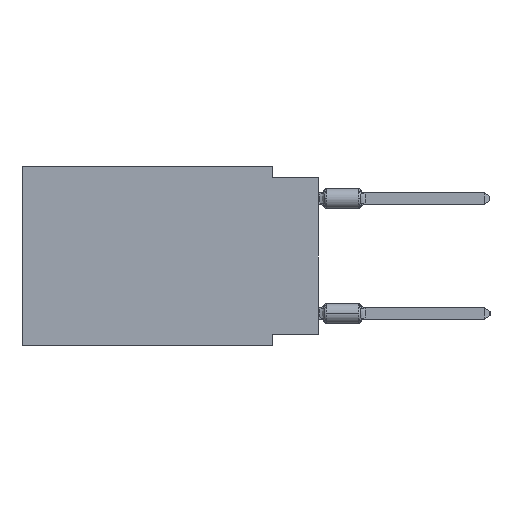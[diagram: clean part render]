
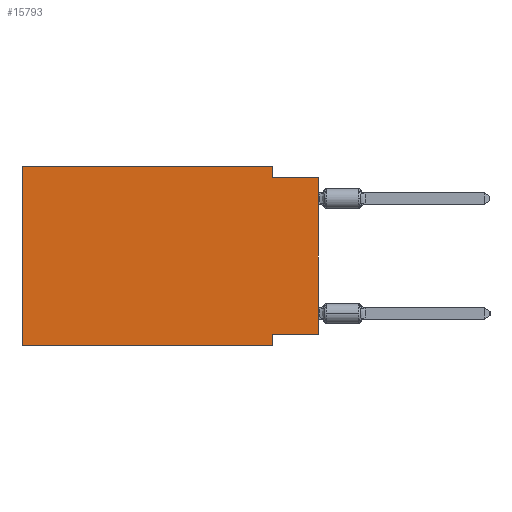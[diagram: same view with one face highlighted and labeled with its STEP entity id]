
A CAD part, left-side view. The second image highlights one B-rep face of the part: STEP entity #15793.
In plain terms, the highlighted planar face has unit normal (-1, 0, 0).
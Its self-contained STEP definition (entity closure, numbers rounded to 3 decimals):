
#2091 = VECTOR ( 'NONE', #58664, 1000. ) ;
#2420 = VECTOR ( 'NONE', #28166, 1000. ) ;
#3125 = VERTEX_POINT ( 'NONE', #43233 ) ;
#4024 = CARTESIAN_POINT ( 'NONE',  ( 0., 16.383, 0. ) ) ;
#6911 = EDGE_CURVE ( 'NONE', #3125, #18494, #40728, .T. ) ;
#9468 = ORIENTED_EDGE ( 'NONE', *, *, #16753, .F. ) ;
#9525 = ORIENTED_EDGE ( 'NONE', *, *, #42792, .T. ) ;
#10156 = ORIENTED_EDGE ( 'NONE', *, *, #6911, .F. ) ;
#11503 = CARTESIAN_POINT ( 'NONE',  ( 0., 2.54, -9.271 ) ) ;
#11882 = CARTESIAN_POINT ( 'NONE',  ( 0., 16.383, 0. ) ) ;
#12308 = VERTEX_POINT ( 'NONE', #44559 ) ;
#12887 = VERTEX_POINT ( 'NONE', #4024 ) ;
#13413 = LINE ( 'NONE', #28790, #2420 ) ;
#13515 = LINE ( 'NONE', #43330, #54010 ) ;
#15793 = ADVANCED_FACE ( 'NONE', ( #32929 ), #52506, .F. ) ;
#16111 = LINE ( 'NONE', #25420, #24041 ) ;
#16753 = EDGE_CURVE ( 'NONE', #30069, #57535, #19929, .T. ) ;
#16764 = AXIS2_PLACEMENT_3D ( 'NONE', #58270, #54104, #39964 ) ;
#18494 = VERTEX_POINT ( 'NONE', #11503 ) ;
#18924 = EDGE_CURVE ( 'NONE', #21496, #30069, #36107, .T. ) ;
#19611 = DIRECTION ( 'NONE',  ( 0., -1., 0. ) ) ;
#19929 = LINE ( 'NONE', #39501, #48427 ) ;
#21496 = VERTEX_POINT ( 'NONE', #26168 ) ;
#23695 = LINE ( 'NONE', #33961, #2091 ) ;
#24041 = VECTOR ( 'NONE', #26359, 1000. ) ;
#25314 = ORIENTED_EDGE ( 'NONE', *, *, #49506, .F. ) ;
#25420 = CARTESIAN_POINT ( 'NONE',  ( 0., 2.54, -9.906 ) ) ;
#26168 = CARTESIAN_POINT ( 'NONE',  ( 0., 2.54, 0. ) ) ;
#26359 = DIRECTION ( 'NONE',  ( 0., 0., -1. ) ) ;
#26451 = EDGE_CURVE ( 'NONE', #12887, #21496, #55822, .T. ) ;
#26794 = ORIENTED_EDGE ( 'NONE', *, *, #26451, .F. ) ;
#28166 = DIRECTION ( 'NONE',  ( 0., -1., 0. ) ) ;
#28790 = CARTESIAN_POINT ( 'NONE',  ( 0., 16.383, -9.906 ) ) ;
#30069 = VERTEX_POINT ( 'NONE', #35934 ) ;
#30843 = ORIENTED_EDGE ( 'NONE', *, *, #46442, .F. ) ;
#31434 = DIRECTION ( 'NONE',  ( 0., -1., 0. ) ) ;
#32929 = FACE_OUTER_BOUND ( 'NONE', #54516, .T. ) ;
#33071 = DIRECTION ( 'NONE',  ( 0., 0., 1. ) ) ;
#33961 = CARTESIAN_POINT ( 'NONE',  ( 0., 0., 0. ) ) ;
#35104 = CARTESIAN_POINT ( 'NONE',  ( 0., 16.383, -9.906 ) ) ;
#35337 = VECTOR ( 'NONE', #31434, 1000. ) ;
#35934 = CARTESIAN_POINT ( 'NONE',  ( 0., 2.54, -0.635 ) ) ;
#36107 = LINE ( 'NONE', #40620, #39380 ) ;
#36393 = EDGE_CURVE ( 'NONE', #3125, #57535, #23695, .T. ) ;
#36430 = ORIENTED_EDGE ( 'NONE', *, *, #18924, .F. ) ;
#39380 = VECTOR ( 'NONE', #55075, 1000. ) ;
#39501 = CARTESIAN_POINT ( 'NONE',  ( 0., 0., -0.635 ) ) ;
#39964 = DIRECTION ( 'NONE',  ( 0., 0., -1. ) ) ;
#40620 = CARTESIAN_POINT ( 'NONE',  ( 0., 2.54, 0. ) ) ;
#40728 = LINE ( 'NONE', #50362, #40956 ) ;
#40956 = VECTOR ( 'NONE', #45854, 1000. ) ;
#42792 = EDGE_CURVE ( 'NONE', #43378, #12308, #13413, .T. ) ;
#43233 = CARTESIAN_POINT ( 'NONE',  ( 0., 0., -9.271 ) ) ;
#43330 = CARTESIAN_POINT ( 'NONE',  ( 0., 16.383, 0. ) ) ;
#43378 = VERTEX_POINT ( 'NONE', #35104 ) ;
#44559 = CARTESIAN_POINT ( 'NONE',  ( 0., 2.54, -9.906 ) ) ;
#45854 = DIRECTION ( 'NONE',  ( 0., 1., 0. ) ) ;
#46442 = EDGE_CURVE ( 'NONE', #43378, #12887, #13515, .T. ) ;
#48427 = VECTOR ( 'NONE', #19611, 1000. ) ;
#49506 = EDGE_CURVE ( 'NONE', #18494, #12308, #16111, .T. ) ;
#50362 = CARTESIAN_POINT ( 'NONE',  ( 0., 0., -9.271 ) ) ;
#51936 = CARTESIAN_POINT ( 'NONE',  ( 0., 0., -0.635 ) ) ;
#52506 = PLANE ( 'NONE',  #16764 ) ;
#54010 = VECTOR ( 'NONE', #33071, 1000. ) ;
#54104 = DIRECTION ( 'NONE',  ( 1., 0., 0. ) ) ;
#54516 = EDGE_LOOP ( 'NONE', ( #63072, #9468, #36430, #26794, #30843, #9525, #25314, #10156 ) ) ;
#55075 = DIRECTION ( 'NONE',  ( 0., 0., -1. ) ) ;
#55822 = LINE ( 'NONE', #11882, #35337 ) ;
#57535 = VERTEX_POINT ( 'NONE', #51936 ) ;
#58270 = CARTESIAN_POINT ( 'NONE',  ( 0., 16.383, 0. ) ) ;
#58664 = DIRECTION ( 'NONE',  ( 0., 0., 1. ) ) ;
#63072 = ORIENTED_EDGE ( 'NONE', *, *, #36393, .T. ) ;
